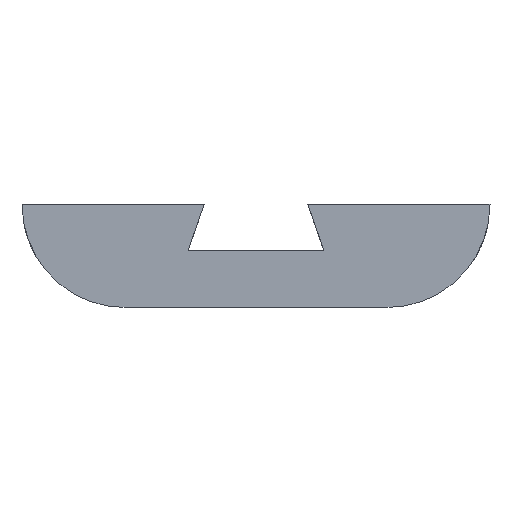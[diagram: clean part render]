
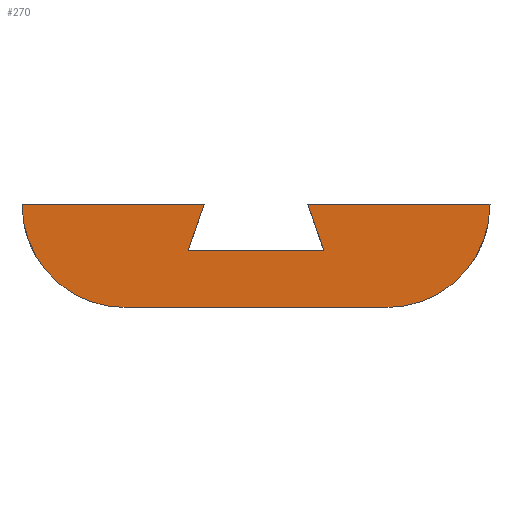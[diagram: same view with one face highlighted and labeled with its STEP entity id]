
A CAD part, front view. The second image highlights one B-rep face of the part: STEP entity #270.
In plain terms, the highlighted planar face has unit normal (0, -1, 0).
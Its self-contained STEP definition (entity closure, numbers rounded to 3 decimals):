
#19=CIRCLE('',#300,8.15);
#20=CIRCLE('',#303,8.15);
#29=PLANE('',#304);
#41=FACE_OUTER_BOUND('',#55,.T.);
#55=EDGE_LOOP('',(#248,#249,#250,#251,#252,#253,#254,#255));
#65=LINE('',#469,#91);
#70=LINE('',#478,#96);
#75=LINE('',#488,#101);
#79=LINE('',#501,#105);
#82=LINE('',#506,#108);
#84=LINE('',#513,#110);
#91=VECTOR('',#324,10.);
#96=VECTOR('',#331,10.);
#101=VECTOR('',#340,10.);
#105=VECTOR('',#352,10.);
#108=VECTOR('',#357,10.);
#110=VECTOR('',#365,10.);
#126=VERTEX_POINT('',#466);
#127=VERTEX_POINT('',#468);
#130=VERTEX_POINT('',#476);
#133=VERTEX_POINT('',#486);
#138=VERTEX_POINT('',#500);
#139=VERTEX_POINT('',#504);
#140=VERTEX_POINT('',#508);
#141=VERTEX_POINT('',#512);
#155=EDGE_CURVE('',#127,#126,#65,.T.);
#160=EDGE_CURVE('',#126,#130,#70,.T.);
#165=EDGE_CURVE('',#130,#133,#75,.T.);
#171=EDGE_CURVE('',#127,#138,#79,.T.);
#174=EDGE_CURVE('',#139,#133,#82,.T.);
#175=EDGE_CURVE('',#140,#139,#19,.T.);
#177=EDGE_CURVE('',#140,#141,#84,.T.);
#179=EDGE_CURVE('',#138,#141,#20,.T.);
#248=ORIENTED_EDGE('',*,*,#165,.T.);
#249=ORIENTED_EDGE('',*,*,#174,.F.);
#250=ORIENTED_EDGE('',*,*,#175,.F.);
#251=ORIENTED_EDGE('',*,*,#177,.T.);
#252=ORIENTED_EDGE('',*,*,#179,.F.);
#253=ORIENTED_EDGE('',*,*,#171,.F.);
#254=ORIENTED_EDGE('',*,*,#155,.T.);
#255=ORIENTED_EDGE('',*,*,#160,.T.);
#270=ADVANCED_FACE('',(#41),#29,.F.);
#300=AXIS2_PLACEMENT_3D('',#509,#360,#361);
#303=AXIS2_PLACEMENT_3D('',#516,#369,#370);
#304=AXIS2_PLACEMENT_3D('',#517,#371,#372);
#324=DIRECTION('',(0.328,0.,-0.945));
#331=DIRECTION('',(-1.,0.,0.));
#340=DIRECTION('',(0.328,0.,0.945));
#352=DIRECTION('',(1.,0.,0.));
#357=DIRECTION('',(1.,0.,0.));
#360=DIRECTION('center_axis',(0.,1.,0.));
#361=DIRECTION('ref_axis',(0.,0.,-1.));
#365=DIRECTION('',(1.,0.,0.));
#369=DIRECTION('center_axis',(0.,1.,0.));
#370=DIRECTION('ref_axis',(1.,0.,0.));
#371=DIRECTION('center_axis',(0.,1.,0.));
#372=DIRECTION('ref_axis',(1.,0.,0.));
#466=CARTESIAN_POINT('',(23.875,0.,4.48));
#468=CARTESIAN_POINT('',(22.6,0.,8.15));
#469=CARTESIAN_POINT('',(23.011,0.,6.967));
#476=CARTESIAN_POINT('',(13.125,0.,4.48));
#478=CARTESIAN_POINT('',(21.188,0.,4.48));
#486=CARTESIAN_POINT('',(14.4,0.,8.15));
#488=CARTESIAN_POINT('',(13.352,0.,5.132));
#500=CARTESIAN_POINT('',(37.,0.,8.15));
#501=CARTESIAN_POINT('',(0.,0.,8.15));
#504=CARTESIAN_POINT('',(0.,0.,8.15));
#506=CARTESIAN_POINT('',(0.,0.,8.15));
#508=CARTESIAN_POINT('',(8.15,0.,0.));
#509=CARTESIAN_POINT('Origin',(8.15,0.,8.15));
#512=CARTESIAN_POINT('',(28.85,0.,0.));
#513=CARTESIAN_POINT('',(0.,0.,0.));
#516=CARTESIAN_POINT('Origin',(28.85,0.,8.15));
#517=CARTESIAN_POINT('Origin',(18.5,0.,4.075));
